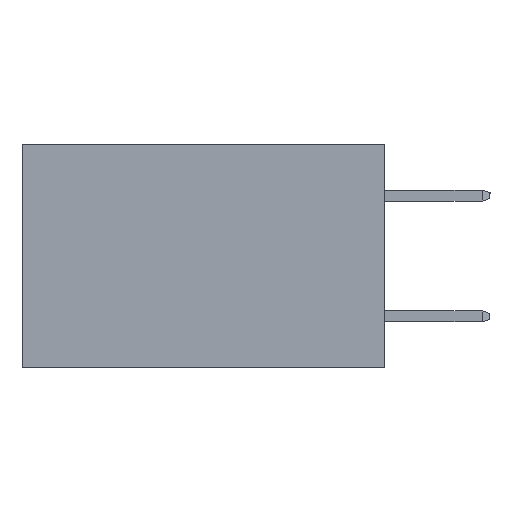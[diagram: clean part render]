
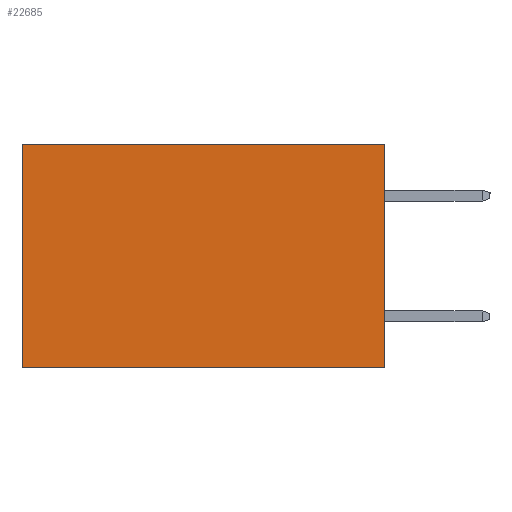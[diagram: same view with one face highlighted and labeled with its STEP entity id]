
A CAD part, left-side view. The second image highlights one B-rep face of the part: STEP entity #22685.
In plain terms, the highlighted planar face has unit normal (-1, 0, 0).
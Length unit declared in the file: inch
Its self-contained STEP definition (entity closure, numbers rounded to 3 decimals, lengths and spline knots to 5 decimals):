
#1352 = EDGE_CURVE ( 'NONE', #7628, #24820, #22999, .T. ) ;
#2000 = VERTEX_POINT ( 'NONE', #24150 ) ;
#3850 = CARTESIAN_POINT ( 'NONE',  ( 0.2615, 0., -0.37 ) ) ;
#4441 = DIRECTION ( 'NONE',  ( 0., 0., -1. ) ) ;
#5062 = CARTESIAN_POINT ( 'NONE',  ( 0.2615, 0., 0. ) ) ;
#5995 = DIRECTION ( 'NONE',  ( 0., 0., -1. ) ) ;
#6565 = LINE ( 'NONE', #19985, #11549 ) ;
#6764 = FACE_OUTER_BOUND ( 'NONE', #10659, .T. ) ;
#7628 = VERTEX_POINT ( 'NONE', #5062 ) ;
#9423 = EDGE_CURVE ( 'NONE', #24820, #22443, #6565, .T. ) ;
#10497 = DIRECTION ( 'NONE',  ( 0., 1., 0. ) ) ;
#10558 = DIRECTION ( 'NONE',  ( 1., 0., 0. ) ) ;
#10659 = EDGE_LOOP ( 'NONE', ( #25106, #12137, #16319, #15632 ) ) ;
#11339 = DIRECTION ( 'NONE',  ( 0., 0., -1. ) ) ;
#11549 = VECTOR ( 'NONE', #10497, 39.37008 ) ;
#11790 = EDGE_CURVE ( 'NONE', #7628, #2000, #24051, .T. ) ;
#12137 = ORIENTED_EDGE ( 'NONE', *, *, #9423, .F. ) ;
#12205 = VECTOR ( 'NONE', #22110, 39.37008 ) ;
#13659 = EDGE_CURVE ( 'NONE', #2000, #22443, #25066, .T. ) ;
#14545 = CARTESIAN_POINT ( 'NONE',  ( 0.2615, 0., -0.37 ) ) ;
#15464 = CARTESIAN_POINT ( 'NONE',  ( 0.2615, 0.6, -0.37 ) ) ;
#15632 = ORIENTED_EDGE ( 'NONE', *, *, #11790, .T. ) ;
#16319 = ORIENTED_EDGE ( 'NONE', *, *, #1352, .F. ) ;
#17144 = CARTESIAN_POINT ( 'NONE',  ( 0.2615, 0.6, -0.37 ) ) ;
#19985 = CARTESIAN_POINT ( 'NONE',  ( 0.2615, 0., -0.37 ) ) ;
#20307 = PLANE ( 'NONE',  #24605 ) ;
#20350 = VECTOR ( 'NONE', #5995, 39.37008 ) ;
#21085 = CARTESIAN_POINT ( 'NONE',  ( 0.2615, 0., -0.37 ) ) ;
#22110 = DIRECTION ( 'NONE',  ( 0., 1., 0. ) ) ;
#22443 = VERTEX_POINT ( 'NONE', #17144 ) ;
#22685 = ADVANCED_FACE ( 'NONE', ( #6764 ), #20307, .F. ) ;
#22999 = LINE ( 'NONE', #21085, #24415 ) ;
#23923 = CARTESIAN_POINT ( 'NONE',  ( 0.2615, 0., 0. ) ) ;
#24051 = LINE ( 'NONE', #23923, #12205 ) ;
#24150 = CARTESIAN_POINT ( 'NONE',  ( 0.2615, 0.6, 0. ) ) ;
#24415 = VECTOR ( 'NONE', #11339, 39.37008 ) ;
#24605 = AXIS2_PLACEMENT_3D ( 'NONE', #14545, #10558, #4441 ) ;
#24820 = VERTEX_POINT ( 'NONE', #3850 ) ;
#25066 = LINE ( 'NONE', #15464, #20350 ) ;
#25106 = ORIENTED_EDGE ( 'NONE', *, *, #13659, .T. ) ;
